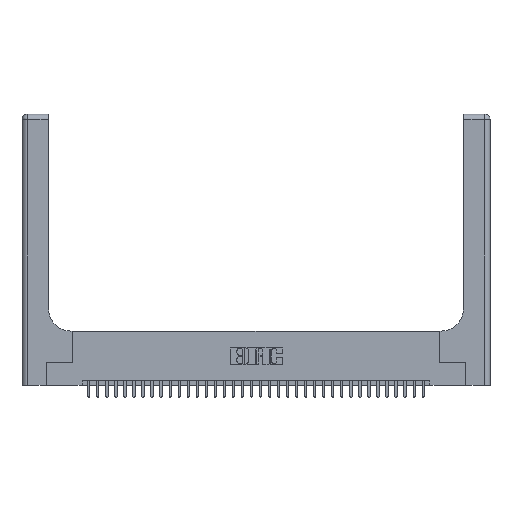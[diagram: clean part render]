
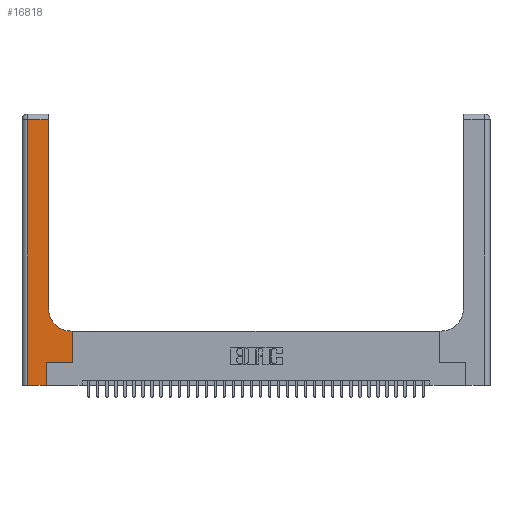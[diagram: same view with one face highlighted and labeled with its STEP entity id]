
A CAD part, top view. The second image highlights one B-rep face of the part: STEP entity #16818.
In plain terms, the highlighted planar face has unit normal (0, 0, 1).
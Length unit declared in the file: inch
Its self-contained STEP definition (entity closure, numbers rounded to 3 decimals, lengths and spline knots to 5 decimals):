
#2151 = CARTESIAN_POINT ( 'NONE',  ( 0.269, 0.25, 0.37 ) ) ;
#2395 = VECTOR ( 'NONE', #8084, 39.37008 ) ;
#2540 = DIRECTION ( 'NONE',  ( 1., 0., 0. ) ) ;
#2625 = CARTESIAN_POINT ( 'NONE',  ( 0., 3., 0.37 ) ) ;
#2776 = ORIENTED_EDGE ( 'NONE', *, *, #13537, .T. ) ;
#2878 = CARTESIAN_POINT ( 'NONE',  ( 0.269, 0., 0.37 ) ) ;
#3071 = VECTOR ( 'NONE', #21789, 39.37008 ) ;
#3531 = CARTESIAN_POINT ( 'NONE',  ( 0., 0., 0.37 ) ) ;
#4040 = CARTESIAN_POINT ( 'NONE',  ( 0.2915, 2.94, 0.37 ) ) ;
#4270 = CARTESIAN_POINT ( 'NONE',  ( 0.2915, 3., 0.37 ) ) ;
#4981 = EDGE_CURVE ( 'NONE', #9947, #12471, #31696, .T. ) ;
#5067 = EDGE_CURVE ( 'NONE', #35179, #6079, #29181, .T. ) ;
#6079 = VERTEX_POINT ( 'NONE', #34535 ) ;
#6340 = ORIENTED_EDGE ( 'NONE', *, *, #9130, .T. ) ;
#7161 = VECTOR ( 'NONE', #30255, 39.37008 ) ;
#8084 = DIRECTION ( 'NONE',  ( 0., -1., 0. ) ) ;
#8143 = VECTOR ( 'NONE', #12704, 39.37008 ) ;
#9130 = EDGE_CURVE ( 'NONE', #21525, #31061, #19557, .T. ) ;
#9193 = EDGE_LOOP ( 'NONE', ( #2776, #11698, #28068, #6340, #29162, #24496, #13358, #24424, #13225 ) ) ;
#9947 = VERTEX_POINT ( 'NONE', #2151 ) ;
#10637 = DIRECTION ( 'NONE',  ( 0., 1., 0. ) ) ;
#10769 = CARTESIAN_POINT ( 'NONE',  ( 0.5415, 0.6, 0.37 ) ) ;
#10982 = PLANE ( 'NONE',  #18548 ) ;
#11016 = CARTESIAN_POINT ( 'NONE',  ( 0., 2.94, 0.37 ) ) ;
#11355 = EDGE_CURVE ( 'NONE', #24822, #13921, #17953, .T. ) ;
#11698 = ORIENTED_EDGE ( 'NONE', *, *, #5067, .T. ) ;
#12471 = VERTEX_POINT ( 'NONE', #29503 ) ;
#12704 = DIRECTION ( 'NONE',  ( 0., 1., 0. ) ) ;
#13225 = ORIENTED_EDGE ( 'NONE', *, *, #11355, .T. ) ;
#13358 = ORIENTED_EDGE ( 'NONE', *, *, #34122, .T. ) ;
#13537 = EDGE_CURVE ( 'NONE', #13921, #35179, #15621, .T. ) ;
#13828 = DIRECTION ( 'NONE',  ( -1., 0., 0. ) ) ;
#13921 = VERTEX_POINT ( 'NONE', #22827 ) ;
#14196 = CARTESIAN_POINT ( 'NONE',  ( 0.269, 0., 0.37 ) ) ;
#14569 = VECTOR ( 'NONE', #16972, 39.37008 ) ;
#15621 = LINE ( 'NONE', #4270, #8143 ) ;
#16818 = ADVANCED_FACE ( 'NONE', ( #34067 ), #10982, .F. ) ;
#16919 = VECTOR ( 'NONE', #10637, 39.37008 ) ;
#16972 = DIRECTION ( 'NONE',  ( 0., 1., 0. ) ) ;
#17193 = LINE ( 'NONE', #27403, #2395 ) ;
#17353 = EDGE_CURVE ( 'NONE', #33331, #24822, #25163, .T. ) ;
#17953 = CIRCLE ( 'NONE', #20287, 0.25 ) ;
#18548 = AXIS2_PLACEMENT_3D ( 'NONE', #2625, #30223, #13828 ) ;
#19146 = CARTESIAN_POINT ( 'NONE',  ( 0.5585, 0.6, 0.37 ) ) ;
#19210 = DIRECTION ( 'NONE',  ( 0., 0., -1. ) ) ;
#19557 = LINE ( 'NONE', #3531, #26817 ) ;
#20287 = AXIS2_PLACEMENT_3D ( 'NONE', #35419, #19210, #2540 ) ;
#21525 = VERTEX_POINT ( 'NONE', #31980 ) ;
#21789 = DIRECTION ( 'NONE',  ( -1., 0., 0. ) ) ;
#21901 = LINE ( 'NONE', #14196, #14569 ) ;
#22827 = CARTESIAN_POINT ( 'NONE',  ( 0.2915, 0.85, 0.37 ) ) ;
#22955 = DIRECTION ( 'NONE',  ( 1., 0., 0. ) ) ;
#23405 = LINE ( 'NONE', #27151, #16919 ) ;
#24424 = ORIENTED_EDGE ( 'NONE', *, *, #17353, .T. ) ;
#24496 = ORIENTED_EDGE ( 'NONE', *, *, #4981, .T. ) ;
#24518 = VECTOR ( 'NONE', #27172, 39.37008 ) ;
#24527 = CARTESIAN_POINT ( 'NONE',  ( 0.2915, 0.6, 0.37 ) ) ;
#24822 = VERTEX_POINT ( 'NONE', #10769 ) ;
#25163 = LINE ( 'NONE', #24527, #3071 ) ;
#26817 = VECTOR ( 'NONE', #22955, 39.37008 ) ;
#27151 = CARTESIAN_POINT ( 'NONE',  ( 0.5585, 0.25, 0.37 ) ) ;
#27172 = DIRECTION ( 'NONE',  ( 1., 0., 0. ) ) ;
#27403 = CARTESIAN_POINT ( 'NONE',  ( 0.06, 3., 0.37 ) ) ;
#28068 = ORIENTED_EDGE ( 'NONE', *, *, #29789, .T. ) ;
#29162 = ORIENTED_EDGE ( 'NONE', *, *, #30297, .T. ) ;
#29181 = LINE ( 'NONE', #11016, #7161 ) ;
#29503 = CARTESIAN_POINT ( 'NONE',  ( 0.5585, 0.25, 0.37 ) ) ;
#29789 = EDGE_CURVE ( 'NONE', #6079, #21525, #17193, .T. ) ;
#30223 = DIRECTION ( 'NONE',  ( 0., 0., -1. ) ) ;
#30255 = DIRECTION ( 'NONE',  ( -1., 0., 0. ) ) ;
#30297 = EDGE_CURVE ( 'NONE', #31061, #9947, #21901, .T. ) ;
#31061 = VERTEX_POINT ( 'NONE', #2878 ) ;
#31696 = LINE ( 'NONE', #32592, #24518 ) ;
#31980 = CARTESIAN_POINT ( 'NONE',  ( 0.06, 0., 0.37 ) ) ;
#32592 = CARTESIAN_POINT ( 'NONE',  ( 0.269, 0.25, 0.37 ) ) ;
#33331 = VERTEX_POINT ( 'NONE', #19146 ) ;
#34067 = FACE_OUTER_BOUND ( 'NONE', #9193, .T. ) ;
#34122 = EDGE_CURVE ( 'NONE', #12471, #33331, #23405, .T. ) ;
#34535 = CARTESIAN_POINT ( 'NONE',  ( 0.06, 2.94, 0.37 ) ) ;
#35179 = VERTEX_POINT ( 'NONE', #4040 ) ;
#35419 = CARTESIAN_POINT ( 'NONE',  ( 0.5415, 0.85, 0.37 ) ) ;
